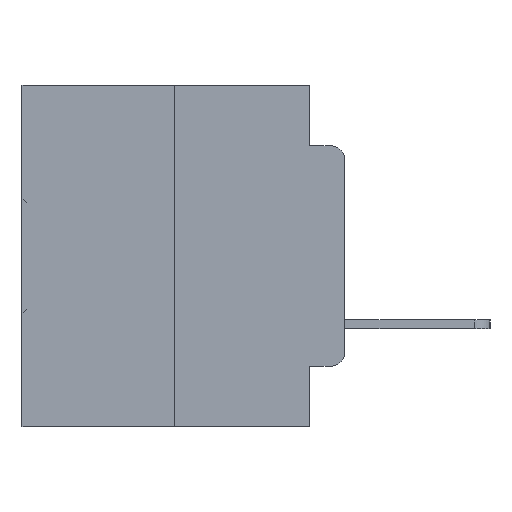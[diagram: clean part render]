
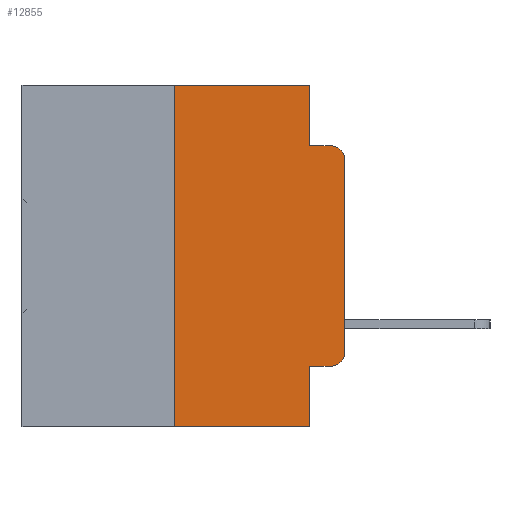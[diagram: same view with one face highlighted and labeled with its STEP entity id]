
A CAD part, left-side view. The second image highlights one B-rep face of the part: STEP entity #12855.
In plain terms, the highlighted planar face has unit normal (-1, 0, 0).
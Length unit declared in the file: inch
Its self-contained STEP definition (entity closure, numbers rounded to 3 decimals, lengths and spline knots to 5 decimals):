
#358 = ORIENTED_EDGE ( 'NONE', *, *, #21245, .F. ) ;
#812 = VERTEX_POINT ( 'NONE', #4815 ) ;
#1145 = DIRECTION ( 'NONE',  ( 1., 0., 0. ) ) ;
#1768 = AXIS2_PLACEMENT_3D ( 'NONE', #7585, #26029, #10293 ) ;
#2255 = VECTOR ( 'NONE', #28157, 39.37008 ) ;
#2306 = DIRECTION ( 'NONE',  ( 0., 0., 1. ) ) ;
#2551 = LINE ( 'NONE', #28870, #15997 ) ;
#2737 = EDGE_CURVE ( 'NONE', #20214, #31627, #6702, .T. ) ;
#3355 = CIRCLE ( 'NONE', #23992, 0.02 ) ;
#4188 = ORIENTED_EDGE ( 'NONE', *, *, #8813, .T. ) ;
#4815 = CARTESIAN_POINT ( 'NONE',  ( 0., 0.25, 0. ) ) ;
#5730 = CARTESIAN_POINT ( 'NONE',  ( 0., 0.02, -0.0885 ) ) ;
#6702 = LINE ( 'NONE', #29499, #27719 ) ;
#7494 = VERTEX_POINT ( 'NONE', #21340 ) ;
#7585 = CARTESIAN_POINT ( 'NONE',  ( 0., 0.02, -0.3915 ) ) ;
#7619 = VECTOR ( 'NONE', #22069, 39.37008 ) ;
#7752 = CARTESIAN_POINT ( 'NONE',  ( 0., 0.051, 0. ) ) ;
#8289 = EDGE_CURVE ( 'NONE', #10848, #18973, #33542, .T. ) ;
#8813 = EDGE_CURVE ( 'NONE', #16974, #33593, #11869, .T. ) ;
#9130 = PLANE ( 'NONE',  #10578 ) ;
#9172 = DIRECTION ( 'NONE',  ( -1., 0., 0. ) ) ;
#9530 = EDGE_CURVE ( 'NONE', #812, #29469, #2551, .T. ) ;
#9603 = ORIENTED_EDGE ( 'NONE', *, *, #10655, .T. ) ;
#9702 = CARTESIAN_POINT ( 'NONE',  ( 0., 0.051, 0. ) ) ;
#10293 = DIRECTION ( 'NONE',  ( 0., 0., -1. ) ) ;
#10578 = AXIS2_PLACEMENT_3D ( 'NONE', #30047, #1145, #19796 ) ;
#10615 = DIRECTION ( 'NONE',  ( 0., -1., 0. ) ) ;
#10655 = EDGE_CURVE ( 'NONE', #33593, #14570, #3355, .T. ) ;
#10848 = VERTEX_POINT ( 'NONE', #12721 ) ;
#11263 = ORIENTED_EDGE ( 'NONE', *, *, #31542, .F. ) ;
#11284 = DIRECTION ( 'NONE',  ( 0., -1., 0. ) ) ;
#11763 = EDGE_CURVE ( 'NONE', #31627, #16974, #33195, .T. ) ;
#11869 = LINE ( 'NONE', #33795, #18910 ) ;
#11953 = CARTESIAN_POINT ( 'NONE',  ( 0., 0.051, -0.5 ) ) ;
#12174 = CARTESIAN_POINT ( 'NONE',  ( 0., 0., -0.1085 ) ) ;
#12721 = CARTESIAN_POINT ( 'NONE',  ( 0., 0.25, -0.5 ) ) ;
#12855 = ADVANCED_FACE ( 'NONE', ( #25272 ), #9130, .F. ) ;
#12903 = VECTOR ( 'NONE', #16967, 39.37008 ) ;
#14570 = VERTEX_POINT ( 'NONE', #5730 ) ;
#14697 = ORIENTED_EDGE ( 'NONE', *, *, #29858, .F. ) ;
#15734 = LINE ( 'NONE', #32581, #21821 ) ;
#15776 = ORIENTED_EDGE ( 'NONE', *, *, #8289, .T. ) ;
#15997 = VECTOR ( 'NONE', #10615, 39.37008 ) ;
#16405 = LINE ( 'NONE', #32252, #7619 ) ;
#16967 = DIRECTION ( 'NONE',  ( 0., -1., 0. ) ) ;
#16974 = VERTEX_POINT ( 'NONE', #29982 ) ;
#18910 = VECTOR ( 'NONE', #2306, 39.37008 ) ;
#18973 = VERTEX_POINT ( 'NONE', #11953 ) ;
#19097 = VECTOR ( 'NONE', #21068, 39.37008 ) ;
#19796 = DIRECTION ( 'NONE',  ( 0., 0., -1. ) ) ;
#19998 = EDGE_LOOP ( 'NONE', ( #4188, #9603, #358, #31457, #33327, #14697, #15776, #11263, #21835, #20628 ) ) ;
#20214 = VERTEX_POINT ( 'NONE', #29856 ) ;
#20628 = ORIENTED_EDGE ( 'NONE', *, *, #11763, .T. ) ;
#21068 = DIRECTION ( 'NONE',  ( 0., -1., 0. ) ) ;
#21245 = EDGE_CURVE ( 'NONE', #7494, #14570, #32735, .T. ) ;
#21340 = CARTESIAN_POINT ( 'NONE',  ( 0., 0.051, -0.0885 ) ) ;
#21821 = VECTOR ( 'NONE', #30147, 39.37008 ) ;
#21835 = ORIENTED_EDGE ( 'NONE', *, *, #2737, .T. ) ;
#22069 = DIRECTION ( 'NONE',  ( 0., 0., -1. ) ) ;
#23014 = EDGE_CURVE ( 'NONE', #29469, #7494, #23475, .T. ) ;
#23475 = LINE ( 'NONE', #9702, #2255 ) ;
#23992 = AXIS2_PLACEMENT_3D ( 'NONE', #25005, #9172, #27545 ) ;
#25005 = CARTESIAN_POINT ( 'NONE',  ( 0., 0.02, -0.1085 ) ) ;
#25272 = FACE_OUTER_BOUND ( 'NONE', #19998, .T. ) ;
#26029 = DIRECTION ( 'NONE',  ( -1., 0., 0. ) ) ;
#27545 = DIRECTION ( 'NONE',  ( 0., 0., -1. ) ) ;
#27598 = CARTESIAN_POINT ( 'NONE',  ( 0., 0.02, -0.4115 ) ) ;
#27719 = VECTOR ( 'NONE', #11284, 39.37008 ) ;
#28157 = DIRECTION ( 'NONE',  ( 0., 0., -1. ) ) ;
#28870 = CARTESIAN_POINT ( 'NONE',  ( 0., 0.473, 0. ) ) ;
#29469 = VERTEX_POINT ( 'NONE', #7752 ) ;
#29499 = CARTESIAN_POINT ( 'NONE',  ( 0., 0.051, -0.4115 ) ) ;
#29856 = CARTESIAN_POINT ( 'NONE',  ( 0., 0.051, -0.4115 ) ) ;
#29858 = EDGE_CURVE ( 'NONE', #10848, #812, #15734, .T. ) ;
#29982 = CARTESIAN_POINT ( 'NONE',  ( 0., 0., -0.3915 ) ) ;
#30047 = CARTESIAN_POINT ( 'NONE',  ( 0., 0.473, 0. ) ) ;
#30147 = DIRECTION ( 'NONE',  ( 0., 0., 1. ) ) ;
#31367 = CARTESIAN_POINT ( 'NONE',  ( 0., 0.051, -0.0885 ) ) ;
#31457 = ORIENTED_EDGE ( 'NONE', *, *, #23014, .F. ) ;
#31542 = EDGE_CURVE ( 'NONE', #20214, #18973, #16405, .T. ) ;
#31627 = VERTEX_POINT ( 'NONE', #27598 ) ;
#32252 = CARTESIAN_POINT ( 'NONE',  ( 0., 0.051, 0. ) ) ;
#32369 = CARTESIAN_POINT ( 'NONE',  ( 0., 0.473, -0.5 ) ) ;
#32581 = CARTESIAN_POINT ( 'NONE',  ( 0., 0.25, 0. ) ) ;
#32735 = LINE ( 'NONE', #31367, #19097 ) ;
#33195 = CIRCLE ( 'NONE', #1768, 0.02 ) ;
#33327 = ORIENTED_EDGE ( 'NONE', *, *, #9530, .F. ) ;
#33542 = LINE ( 'NONE', #32369, #12903 ) ;
#33593 = VERTEX_POINT ( 'NONE', #12174 ) ;
#33795 = CARTESIAN_POINT ( 'NONE',  ( 0., 0., 0. ) ) ;
